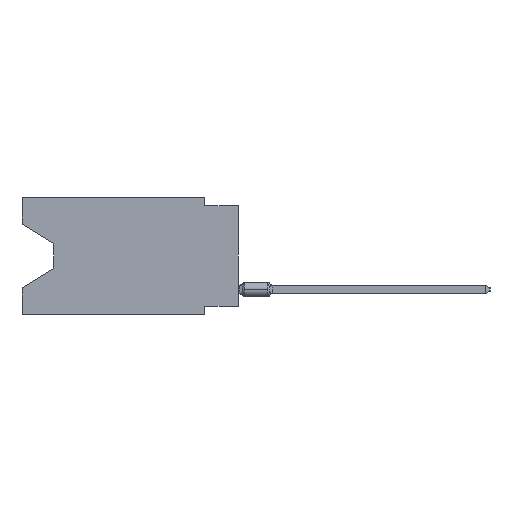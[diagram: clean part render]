
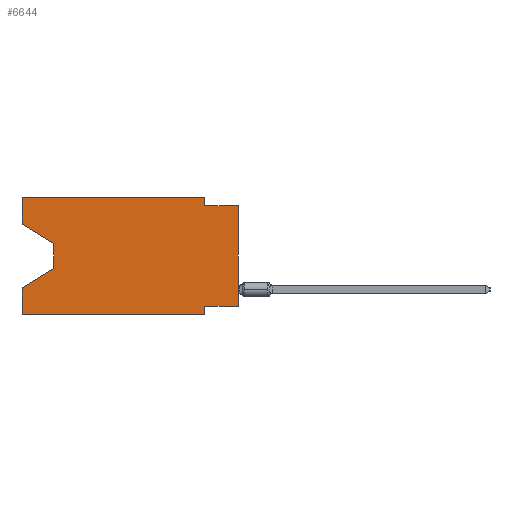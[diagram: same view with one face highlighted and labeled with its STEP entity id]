
A CAD part, left-side view. The second image highlights one B-rep face of the part: STEP entity #6644.
In plain terms, the highlighted planar face has unit normal (-1, 0, 0).
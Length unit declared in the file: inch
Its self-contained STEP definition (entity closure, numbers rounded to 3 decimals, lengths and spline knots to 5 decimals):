
#228 = CARTESIAN_POINT ( 'NONE',  ( 0., 0., -0.025 ) ) ;
#397 = LINE ( 'NONE', #29475, #2508 ) ;
#1289 = VERTEX_POINT ( 'NONE', #23586 ) ;
#1384 = DIRECTION ( 'NONE',  ( 0., 0., -1. ) ) ;
#1886 = EDGE_CURVE ( 'NONE', #41355, #46555, #7800, .T. ) ;
#1905 = FACE_OUTER_BOUND ( 'NONE', #21477, .T. ) ;
#2508 = VECTOR ( 'NONE', #5287, 39.37008 ) ;
#2558 = LINE ( 'NONE', #43822, #6650 ) ;
#2632 = VECTOR ( 'NONE', #41102, 39.37008 ) ;
#2828 = EDGE_CURVE ( 'NONE', #8321, #37907, #45856, .T. ) ;
#3300 = CARTESIAN_POINT ( 'NONE',  ( 0., 0.645, -0.35 ) ) ;
#4450 = LINE ( 'NONE', #20767, #2632 ) ;
#5260 = LINE ( 'NONE', #30239, #24417 ) ;
#5287 = DIRECTION ( 'NONE',  ( 0., 0., -1. ) ) ;
#5712 = DIRECTION ( 'NONE',  ( 0., 0., -1. ) ) ;
#5985 = ORIENTED_EDGE ( 'NONE', *, *, #47355, .F. ) ;
#6623 = DIRECTION ( 'NONE',  ( 0., -1., 0. ) ) ;
#6644 = ADVANCED_FACE ( 'NONE', ( #1905 ), #34513, .F. ) ;
#6650 = VECTOR ( 'NONE', #6623, 39.37008 ) ;
#7800 = LINE ( 'NONE', #36854, #17681 ) ;
#8116 = VERTEX_POINT ( 'NONE', #3300 ) ;
#8321 = VERTEX_POINT ( 'NONE', #34253 ) ;
#8423 = LINE ( 'NONE', #20404, #23910 ) ;
#9013 = LINE ( 'NONE', #34018, #29466 ) ;
#10439 = EDGE_CURVE ( 'NONE', #41355, #52769, #53033, .T. ) ;
#10588 = CARTESIAN_POINT ( 'NONE',  ( 0., 0.1, 0. ) ) ;
#11069 = EDGE_CURVE ( 'NONE', #52777, #1289, #21799, .T. ) ;
#11379 = VECTOR ( 'NONE', #16537, 39.37008 ) ;
#11935 = ORIENTED_EDGE ( 'NONE', *, *, #13228, .F. ) ;
#12170 = CARTESIAN_POINT ( 'NONE',  ( 0., 0.55, -0.212 ) ) ;
#12547 = DIRECTION ( 'NONE',  ( 0., 0., -1. ) ) ;
#13119 = ORIENTED_EDGE ( 'NONE', *, *, #34614, .T. ) ;
#13228 = EDGE_CURVE ( 'NONE', #46555, #39663, #4450, .T. ) ;
#13276 = CARTESIAN_POINT ( 'NONE',  ( 0., 0.645, -0.08025 ) ) ;
#13342 = CARTESIAN_POINT ( 'NONE',  ( 0., 0.645, 0. ) ) ;
#13865 = VECTOR ( 'NONE', #28575, 39.37008 ) ;
#14145 = VECTOR ( 'NONE', #38003, 39.37008 ) ;
#14342 = ORIENTED_EDGE ( 'NONE', *, *, #11069, .F. ) ;
#14382 = CARTESIAN_POINT ( 'NONE',  ( 0., 0., -0.325 ) ) ;
#16537 = DIRECTION ( 'NONE',  ( 0., -1., 0. ) ) ;
#17681 = VECTOR ( 'NONE', #36593, 39.37008 ) ;
#19243 = ORIENTED_EDGE ( 'NONE', *, *, #24398, .T. ) ;
#20404 = CARTESIAN_POINT ( 'NONE',  ( 0., 0.645, 0. ) ) ;
#20489 = CARTESIAN_POINT ( 'NONE',  ( 0., 0.645, -0.26975 ) ) ;
#20767 = CARTESIAN_POINT ( 'NONE',  ( 0., 0.645, 0. ) ) ;
#21477 = EDGE_LOOP ( 'NONE', ( #40885, #19243, #40198, #5985, #13119, #14342, #45971, #46760, #36111, #23308, #11935, #44049 ) ) ;
#21799 = LINE ( 'NONE', #42402, #39777 ) ;
#23308 = ORIENTED_EDGE ( 'NONE', *, *, #48314, .F. ) ;
#23586 = CARTESIAN_POINT ( 'NONE',  ( 0., 0.1, -0.35 ) ) ;
#23847 = CARTESIAN_POINT ( 'NONE',  ( 0., 0.645, 0. ) ) ;
#23910 = VECTOR ( 'NONE', #53524, 39.37008 ) ;
#24398 = EDGE_CURVE ( 'NONE', #52769, #29146, #9013, .T. ) ;
#24417 = VECTOR ( 'NONE', #49799, 39.37008 ) ;
#26093 = VERTEX_POINT ( 'NONE', #48474 ) ;
#28575 = DIRECTION ( 'NONE',  ( 0., -0.855, -0.519 ) ) ;
#29100 = CARTESIAN_POINT ( 'NONE',  ( 0., 0.55, -0.138 ) ) ;
#29146 = VERTEX_POINT ( 'NONE', #12170 ) ;
#29466 = VECTOR ( 'NONE', #12547, 39.37008 ) ;
#29475 = CARTESIAN_POINT ( 'NONE',  ( 0., 0.1, 0. ) ) ;
#29914 = DIRECTION ( 'NONE',  ( 1., 0., 0. ) ) ;
#30051 = AXIS2_PLACEMENT_3D ( 'NONE', #13342, #29914, #5712 ) ;
#30239 = CARTESIAN_POINT ( 'NONE',  ( 0., 0.55, -0.212 ) ) ;
#31944 = VECTOR ( 'NONE', #33778, 39.37008 ) ;
#32303 = CARTESIAN_POINT ( 'NONE',  ( 0., 0.645, -0.08025 ) ) ;
#33181 = CARTESIAN_POINT ( 'NONE',  ( 0., 0.1, -0.325 ) ) ;
#33778 = DIRECTION ( 'NONE',  ( 0., 1., 0. ) ) ;
#34018 = CARTESIAN_POINT ( 'NONE',  ( 0., 0.55, -0.138 ) ) ;
#34253 = CARTESIAN_POINT ( 'NONE',  ( 0., 0., -0.325 ) ) ;
#34513 = PLANE ( 'NONE',  #30051 ) ;
#34614 = EDGE_CURVE ( 'NONE', #8116, #1289, #2558, .T. ) ;
#35371 = CARTESIAN_POINT ( 'NONE',  ( 0., 0., -0.025 ) ) ;
#36111 = ORIENTED_EDGE ( 'NONE', *, *, #41524, .F. ) ;
#36495 = EDGE_CURVE ( 'NONE', #8321, #52777, #50335, .T. ) ;
#36593 = DIRECTION ( 'NONE',  ( 0., 0., 1. ) ) ;
#36854 = CARTESIAN_POINT ( 'NONE',  ( 0., 0.645, 0. ) ) ;
#37172 = LINE ( 'NONE', #228, #11379 ) ;
#37907 = VERTEX_POINT ( 'NONE', #35371 ) ;
#38003 = DIRECTION ( 'NONE',  ( 0., 0., 1. ) ) ;
#39663 = VERTEX_POINT ( 'NONE', #10588 ) ;
#39777 = VECTOR ( 'NONE', #1384, 39.37008 ) ;
#40198 = ORIENTED_EDGE ( 'NONE', *, *, #52436, .T. ) ;
#40394 = VERTEX_POINT ( 'NONE', #20489 ) ;
#40885 = ORIENTED_EDGE ( 'NONE', *, *, #10439, .T. ) ;
#41102 = DIRECTION ( 'NONE',  ( 0., -1., 0. ) ) ;
#41355 = VERTEX_POINT ( 'NONE', #32303 ) ;
#41524 = EDGE_CURVE ( 'NONE', #26093, #37907, #37172, .T. ) ;
#42402 = CARTESIAN_POINT ( 'NONE',  ( 0., 0.1, -0.35 ) ) ;
#43822 = CARTESIAN_POINT ( 'NONE',  ( 0., 0.645, -0.35 ) ) ;
#44049 = ORIENTED_EDGE ( 'NONE', *, *, #1886, .F. ) ;
#45856 = LINE ( 'NONE', #49951, #14145 ) ;
#45971 = ORIENTED_EDGE ( 'NONE', *, *, #36495, .F. ) ;
#46555 = VERTEX_POINT ( 'NONE', #23847 ) ;
#46760 = ORIENTED_EDGE ( 'NONE', *, *, #2828, .T. ) ;
#47355 = EDGE_CURVE ( 'NONE', #8116, #40394, #8423, .T. ) ;
#48314 = EDGE_CURVE ( 'NONE', #39663, #26093, #397, .T. ) ;
#48474 = CARTESIAN_POINT ( 'NONE',  ( 0., 0.1, -0.025 ) ) ;
#49799 = DIRECTION ( 'NONE',  ( 0., 0.855, -0.519 ) ) ;
#49951 = CARTESIAN_POINT ( 'NONE',  ( 0., 0., 0. ) ) ;
#50335 = LINE ( 'NONE', #14382, #31944 ) ;
#52436 = EDGE_CURVE ( 'NONE', #29146, #40394, #5260, .T. ) ;
#52769 = VERTEX_POINT ( 'NONE', #29100 ) ;
#52777 = VERTEX_POINT ( 'NONE', #33181 ) ;
#53033 = LINE ( 'NONE', #13276, #13865 ) ;
#53524 = DIRECTION ( 'NONE',  ( 0., 0., 1. ) ) ;
